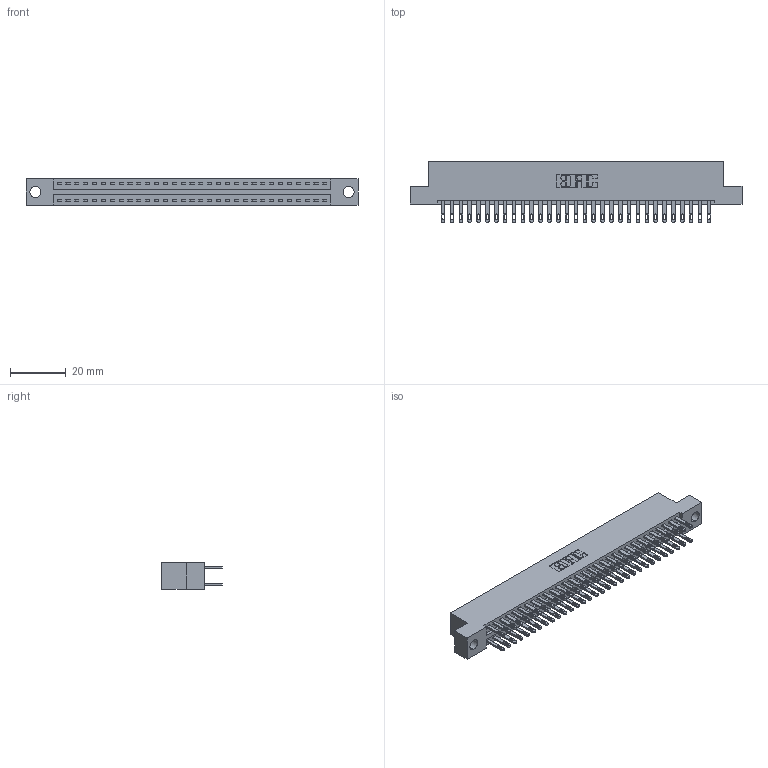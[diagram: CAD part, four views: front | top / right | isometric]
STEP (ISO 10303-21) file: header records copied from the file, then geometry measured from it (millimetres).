
FILE_DESCRIPTION (( 'STEP AP203' ), '1' );
FILE_NAME ('896-062-500-204.STEP', '2021-07-28T00:32:11', ( '' ), ( '' ), 'SwSTEP 2.0', 'SolidWorks 2020', '' );
FILE_SCHEMA (( 'CONFIG_CONTROL_DESIGN' ));
Length unit declared in the file: inch
Products named in the file (3): 345-292-001_345-293-100; 896-062-500-204; 846 Part_Flush Mounting Lugs - 0.156 Dia-TH
Assembly tree (63 placements, depth 2):
  896-062-500-204
    846 Part_Flush Mounting Lugs - 0.156 Dia-TH
    345-292-001_345-293-100  x62
Bounding box: 119 x 21.84 x 9.4 mm (x, y, z)
Volume: 11620.1 mm3; surface area: 16261.9 mm2
Topology: 63 solids, 63 shells, 3098 faces, 9443 edges, 6294 vertices
Faces by surface type: plane 1874, cylinder 1224
Entity records: 21645 total; most frequent: CARTESIAN_POINT 3580, ORIENTED_EDGE 3514, DIRECTION 3209, EDGE_CURVE 1757, VECTOR 1497, LINE 1497, VERTEX_POINT 1170, AXIS2_PLACEMENT_3D 856
